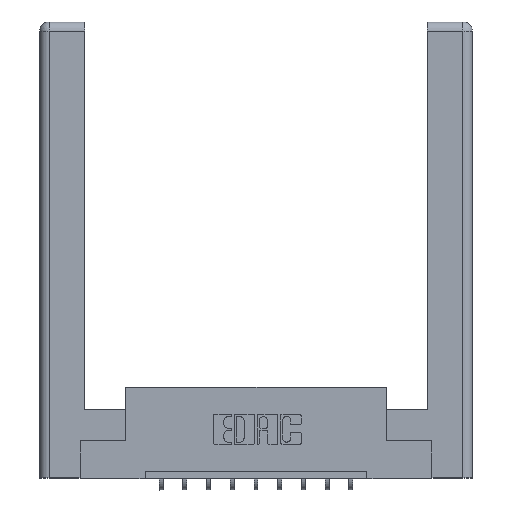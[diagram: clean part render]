
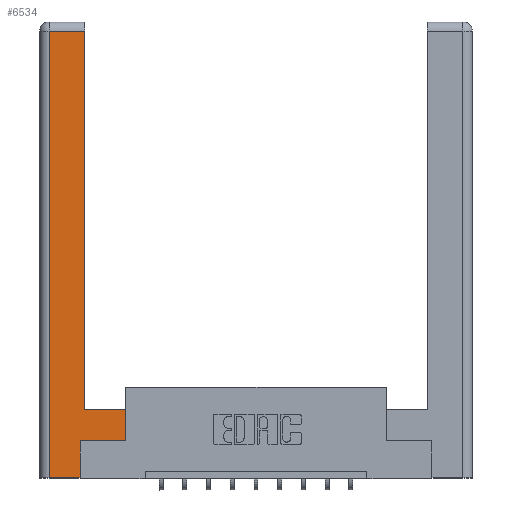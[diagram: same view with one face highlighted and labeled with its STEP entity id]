
A CAD part, top view. The second image highlights one B-rep face of the part: STEP entity #6534.
In plain terms, the highlighted planar face has unit normal (0, 0, 1).
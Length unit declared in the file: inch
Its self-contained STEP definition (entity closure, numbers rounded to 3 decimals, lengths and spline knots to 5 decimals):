
#16 = ORIENTED_EDGE ( 'NONE', *, *, #9762, .T. ) ;
#323 = EDGE_CURVE ( 'NONE', #1405, #5617, #491, .T. ) ;
#491 = LINE ( 'NONE', #12116, #3602 ) ;
#816 = DIRECTION ( 'NONE',  ( -1., 0., 0. ) ) ;
#986 = LINE ( 'NONE', #8908, #6221 ) ;
#1006 = CARTESIAN_POINT ( 'NONE',  ( 0.565, 0.45, 0. ) ) ;
#1102 = LINE ( 'NONE', #11983, #9202 ) ;
#1348 = ORIENTED_EDGE ( 'NONE', *, *, #323, .T. ) ;
#1405 = VERTEX_POINT ( 'NONE', #6122 ) ;
#1535 = AXIS2_PLACEMENT_3D ( 'NONE', #8303, #10302, #9389 ) ;
#2386 = ORIENTED_EDGE ( 'NONE', *, *, #7434, .T. ) ;
#2738 = CARTESIAN_POINT ( 'NONE',  ( 0.265, 0.245, 0. ) ) ;
#2949 = LINE ( 'NONE', #3665, #5898 ) ;
#3055 = ORIENTED_EDGE ( 'NONE', *, *, #9991, .T. ) ;
#3602 = VECTOR ( 'NONE', #4756, 39.37008 ) ;
#3665 = CARTESIAN_POINT ( 'NONE',  ( 0.265, 0.245, 0. ) ) ;
#3760 = ORIENTED_EDGE ( 'NONE', *, *, #8377, .T. ) ;
#3822 = ORIENTED_EDGE ( 'NONE', *, *, #6456, .T. ) ;
#3974 = LINE ( 'NONE', #10484, #9626 ) ;
#4066 = LINE ( 'NONE', #9091, #12219 ) ;
#4679 = CARTESIAN_POINT ( 'NONE',  ( 0.0615, 2.94, 0. ) ) ;
#4745 = VECTOR ( 'NONE', #816, 39.37008 ) ;
#4756 = DIRECTION ( 'NONE',  ( 1., 0., 0. ) ) ;
#4908 = VERTEX_POINT ( 'NONE', #12111 ) ;
#5061 = FACE_OUTER_BOUND ( 'NONE', #7245, .T. ) ;
#5114 = CARTESIAN_POINT ( 'NONE',  ( 0.565, 0.45, 0. ) ) ;
#5503 = CARTESIAN_POINT ( 'NONE',  ( 0.265, 0., 0. ) ) ;
#5617 = VERTEX_POINT ( 'NONE', #5503 ) ;
#5898 = VECTOR ( 'NONE', #12211, 39.37008 ) ;
#5912 = DIRECTION ( 'NONE',  ( 1., 0., 0. ) ) ;
#6070 = CARTESIAN_POINT ( 'NONE',  ( 0.295, 2.94, 0. ) ) ;
#6122 = CARTESIAN_POINT ( 'NONE',  ( 0.0615, 0., 0. ) ) ;
#6221 = VECTOR ( 'NONE', #8859, 39.37008 ) ;
#6367 = ORIENTED_EDGE ( 'NONE', *, *, #10014, .T. ) ;
#6456 = EDGE_CURVE ( 'NONE', #8979, #1405, #986, .T. ) ;
#6534 = ADVANCED_FACE ( 'NONE', ( #5061 ), #7231, .F. ) ;
#6710 = DIRECTION ( 'NONE',  ( -1., 0., 0. ) ) ;
#7231 = PLANE ( 'NONE',  #1535 ) ;
#7245 = EDGE_LOOP ( 'NONE', ( #9849, #16, #3822, #1348, #6367, #2386, #3055, #3760 ) ) ;
#7434 = EDGE_CURVE ( 'NONE', #9150, #4908, #4066, .T. ) ;
#7821 = DIRECTION ( 'NONE',  ( 0., 1., 0. ) ) ;
#7999 = VERTEX_POINT ( 'NONE', #12228 ) ;
#8303 = CARTESIAN_POINT ( 'NONE',  ( 0., 0., 0. ) ) ;
#8377 = EDGE_CURVE ( 'NONE', #13124, #7999, #1102, .T. ) ;
#8859 = DIRECTION ( 'NONE',  ( 0., -1., 0. ) ) ;
#8908 = CARTESIAN_POINT ( 'NONE',  ( 0.0615, 0., 0. ) ) ;
#8979 = VERTEX_POINT ( 'NONE', #11083 ) ;
#9091 = CARTESIAN_POINT ( 'NONE',  ( 0.565, 0.245, 0. ) ) ;
#9150 = VERTEX_POINT ( 'NONE', #2738 ) ;
#9202 = VECTOR ( 'NONE', #6710, 39.37008 ) ;
#9349 = DIRECTION ( 'NONE',  ( 0., 1., 0. ) ) ;
#9389 = DIRECTION ( 'NONE',  ( -1., 0., 0. ) ) ;
#9626 = VECTOR ( 'NONE', #9349, 39.37008 ) ;
#9732 = VECTOR ( 'NONE', #7821, 39.37008 ) ;
#9762 = EDGE_CURVE ( 'NONE', #9984, #8979, #12893, .T. ) ;
#9849 = ORIENTED_EDGE ( 'NONE', *, *, #13663, .T. ) ;
#9984 = VERTEX_POINT ( 'NONE', #6070 ) ;
#9991 = EDGE_CURVE ( 'NONE', #4908, #13124, #12561, .T. ) ;
#10014 = EDGE_CURVE ( 'NONE', #5617, #9150, #2949, .T. ) ;
#10302 = DIRECTION ( 'NONE',  ( 0., 0., -1. ) ) ;
#10484 = CARTESIAN_POINT ( 'NONE',  ( 0.295, 3., 0. ) ) ;
#11083 = CARTESIAN_POINT ( 'NONE',  ( 0.0615, 2.94, 0. ) ) ;
#11983 = CARTESIAN_POINT ( 'NONE',  ( 0.295, 0.45, 0. ) ) ;
#12111 = CARTESIAN_POINT ( 'NONE',  ( 0.565, 0.245, 0. ) ) ;
#12116 = CARTESIAN_POINT ( 'NONE',  ( 0.265, 0., 0. ) ) ;
#12211 = DIRECTION ( 'NONE',  ( 0., 1., 0. ) ) ;
#12219 = VECTOR ( 'NONE', #5912, 39.37008 ) ;
#12228 = CARTESIAN_POINT ( 'NONE',  ( 0.295, 0.45, 0. ) ) ;
#12561 = LINE ( 'NONE', #5114, #9732 ) ;
#12893 = LINE ( 'NONE', #4679, #4745 ) ;
#13124 = VERTEX_POINT ( 'NONE', #1006 ) ;
#13663 = EDGE_CURVE ( 'NONE', #7999, #9984, #3974, .T. ) ;
